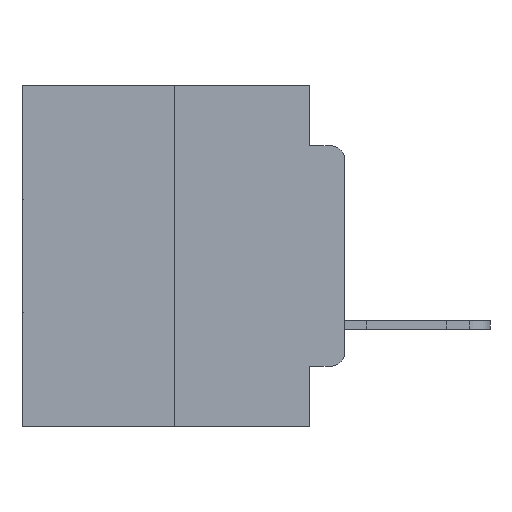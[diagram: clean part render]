
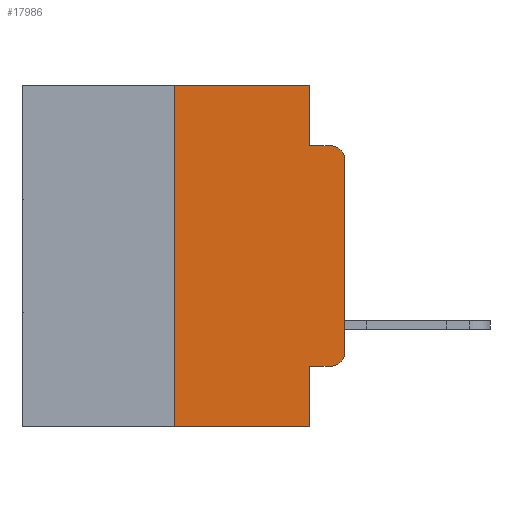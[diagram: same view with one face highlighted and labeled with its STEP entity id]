
A CAD part, left-side view. The second image highlights one B-rep face of the part: STEP entity #17986.
In plain terms, the highlighted planar face has unit normal (-1, 0, 0).
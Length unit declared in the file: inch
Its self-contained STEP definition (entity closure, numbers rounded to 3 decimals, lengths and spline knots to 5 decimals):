
#201 = ORIENTED_EDGE ( 'NONE', *, *, #24162, .T. ) ;
#263 = ORIENTED_EDGE ( 'NONE', *, *, #24190, .F. ) ;
#564 = LINE ( 'NONE', #11556, #28308 ) ;
#1340 = ORIENTED_EDGE ( 'NONE', *, *, #24195, .F. ) ;
#1909 = DIRECTION ( 'NONE',  ( 0., 0., -1. ) ) ;
#2195 = DIRECTION ( 'NONE',  ( 0., -1., 0. ) ) ;
#2341 = ORIENTED_EDGE ( 'NONE', *, *, #9637, .F. ) ;
#2817 = ORIENTED_EDGE ( 'NONE', *, *, #24231, .F. ) ;
#2896 = CARTESIAN_POINT ( 'NONE',  ( 0., 0.473, 0. ) ) ;
#3042 = CARTESIAN_POINT ( 'NONE',  ( 0., 0.473, -0.5 ) ) ;
#3188 = VERTEX_POINT ( 'NONE', #17003 ) ;
#3549 = VERTEX_POINT ( 'NONE', #27134 ) ;
#3758 = ORIENTED_EDGE ( 'NONE', *, *, #21995, .T. ) ;
#4157 = CIRCLE ( 'NONE', #13890, 0.02 ) ;
#4372 = VERTEX_POINT ( 'NONE', #6669 ) ;
#4399 = LINE ( 'NONE', #2896, #20974 ) ;
#4953 = ORIENTED_EDGE ( 'NONE', *, *, #24234, .F. ) ;
#5728 = LINE ( 'NONE', #13950, #11150 ) ;
#6669 = CARTESIAN_POINT ( 'NONE',  ( 0., 0.051, 0. ) ) ;
#7943 = CIRCLE ( 'NONE', #10833, 0.02 ) ;
#8651 = LINE ( 'NONE', #26086, #25214 ) ;
#8948 = DIRECTION ( 'NONE',  ( 0., 0., 1. ) ) ;
#9230 = DIRECTION ( 'NONE',  ( 0., -1., 0. ) ) ;
#9460 = ORIENTED_EDGE ( 'NONE', *, *, #24239, .T. ) ;
#9525 = CARTESIAN_POINT ( 'NONE',  ( 0., 0.02, -0.3915 ) ) ;
#9637 = EDGE_CURVE ( 'NONE', #3549, #4372, #4399, .T. ) ;
#10701 = EDGE_LOOP ( 'NONE', ( #20881, #201, #263, #1340, #2341, #2817, #3758, #4953, #9460, #11408 ) ) ;
#10833 = AXIS2_PLACEMENT_3D ( 'NONE', #28039, #16029, #1909 ) ;
#11150 = VECTOR ( 'NONE', #16209, 39.37008 ) ;
#11408 = ORIENTED_EDGE ( 'NONE', *, *, #24266, .T. ) ;
#11556 = CARTESIAN_POINT ( 'NONE',  ( 0., 0.051, 0. ) ) ;
#11854 = DIRECTION ( 'NONE',  ( 0., 0., -1. ) ) ;
#12565 = VECTOR ( 'NONE', #9230, 39.37008 ) ;
#13302 = LINE ( 'NONE', #22403, #12565 ) ;
#13464 = CARTESIAN_POINT ( 'NONE',  ( 0., 0.051, -0.0885 ) ) ;
#13851 = DIRECTION ( 'NONE',  ( 0., 0., -1. ) ) ;
#13890 = AXIS2_PLACEMENT_3D ( 'NONE', #9525, #24671, #11854 ) ;
#13950 = CARTESIAN_POINT ( 'NONE',  ( 0., 0.051, 0. ) ) ;
#14369 = VERTEX_POINT ( 'NONE', #17887 ) ;
#14499 = VERTEX_POINT ( 'NONE', #13464 ) ;
#15521 = DIRECTION ( 'NONE',  ( 0., 0., -1. ) ) ;
#15574 = CARTESIAN_POINT ( 'NONE',  ( 0., 0.051, -0.4115 ) ) ;
#15615 = DIRECTION ( 'NONE',  ( 1., 0., 0. ) ) ;
#15903 = CARTESIAN_POINT ( 'NONE',  ( 0., 0.473, 0. ) ) ;
#16029 = DIRECTION ( 'NONE',  ( -1., 0., 0. ) ) ;
#16044 = PLANE ( 'NONE',  #16172 ) ;
#16172 = AXIS2_PLACEMENT_3D ( 'NONE', #15903, #15615, #15521 ) ;
#16209 = DIRECTION ( 'NONE',  ( 0., 0., -1. ) ) ;
#16929 = CARTESIAN_POINT ( 'NONE',  ( 0., 0.25, -0.5 ) ) ;
#17003 = CARTESIAN_POINT ( 'NONE',  ( 0., 0., -0.1085 ) ) ;
#17887 = CARTESIAN_POINT ( 'NONE',  ( 0., 0., -0.3915 ) ) ;
#17986 = ADVANCED_FACE ( 'NONE', ( #23473 ), #16044, .F. ) ;
#18343 = CARTESIAN_POINT ( 'NONE',  ( 0., 0.051, -0.4115 ) ) ;
#18401 = VERTEX_POINT ( 'NONE', #24514 ) ;
#18447 = VECTOR ( 'NONE', #26399, 39.37008 ) ;
#20134 = VERTEX_POINT ( 'NONE', #15574 ) ;
#20339 = VERTEX_POINT ( 'NONE', #26734 ) ;
#20463 = VERTEX_POINT ( 'NONE', #25359 ) ;
#20495 = DIRECTION ( 'NONE',  ( 0., -1., 0. ) ) ;
#20881 = ORIENTED_EDGE ( 'NONE', *, *, #24088, .T. ) ;
#20974 = VECTOR ( 'NONE', #2195, 39.37008 ) ;
#21546 = VECTOR ( 'NONE', #23303, 39.37008 ) ;
#21995 = EDGE_CURVE ( 'NONE', #24482, #20463, #26738, .T. ) ;
#22087 = VECTOR ( 'NONE', #20495, 39.37008 ) ;
#22403 = CARTESIAN_POINT ( 'NONE',  ( 0., 0.051, -0.0885 ) ) ;
#22745 = LINE ( 'NONE', #18343, #22087 ) ;
#23303 = DIRECTION ( 'NONE',  ( 0., -1., 0. ) ) ;
#23355 = LINE ( 'NONE', #24496, #18447 ) ;
#23473 = FACE_OUTER_BOUND ( 'NONE', #10701, .T. ) ;
#24088 = EDGE_CURVE ( 'NONE', #14369, #3188, #8651, .T. ) ;
#24162 = EDGE_CURVE ( 'NONE', #3188, #20339, #7943, .T. ) ;
#24190 = EDGE_CURVE ( 'NONE', #14499, #20339, #13302, .T. ) ;
#24195 = EDGE_CURVE ( 'NONE', #4372, #14499, #564, .T. ) ;
#24231 = EDGE_CURVE ( 'NONE', #24482, #3549, #23355, .T. ) ;
#24234 = EDGE_CURVE ( 'NONE', #20134, #20463, #5728, .T. ) ;
#24239 = EDGE_CURVE ( 'NONE', #20134, #18401, #22745, .T. ) ;
#24266 = EDGE_CURVE ( 'NONE', #18401, #14369, #4157, .T. ) ;
#24482 = VERTEX_POINT ( 'NONE', #16929 ) ;
#24496 = CARTESIAN_POINT ( 'NONE',  ( 0., 0.25, 0. ) ) ;
#24514 = CARTESIAN_POINT ( 'NONE',  ( 0., 0.02, -0.4115 ) ) ;
#24671 = DIRECTION ( 'NONE',  ( -1., 0., 0. ) ) ;
#25214 = VECTOR ( 'NONE', #8948, 39.37008 ) ;
#25359 = CARTESIAN_POINT ( 'NONE',  ( 0., 0.051, -0.5 ) ) ;
#26086 = CARTESIAN_POINT ( 'NONE',  ( 0., 0., 0. ) ) ;
#26399 = DIRECTION ( 'NONE',  ( 0., 0., 1. ) ) ;
#26734 = CARTESIAN_POINT ( 'NONE',  ( 0., 0.02, -0.0885 ) ) ;
#26738 = LINE ( 'NONE', #3042, #21546 ) ;
#27134 = CARTESIAN_POINT ( 'NONE',  ( 0., 0.25, 0. ) ) ;
#28039 = CARTESIAN_POINT ( 'NONE',  ( 0., 0.02, -0.1085 ) ) ;
#28308 = VECTOR ( 'NONE', #13851, 39.37008 ) ;
